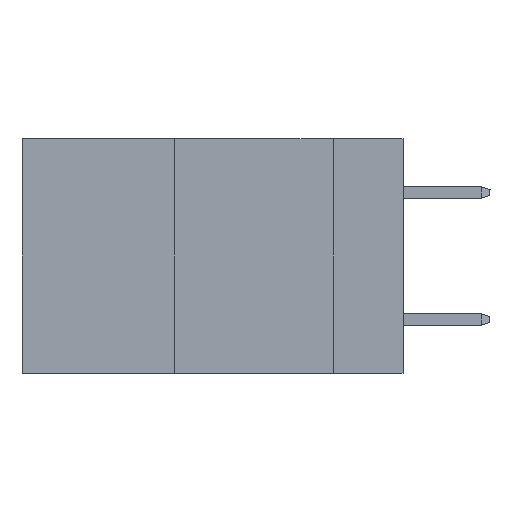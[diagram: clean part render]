
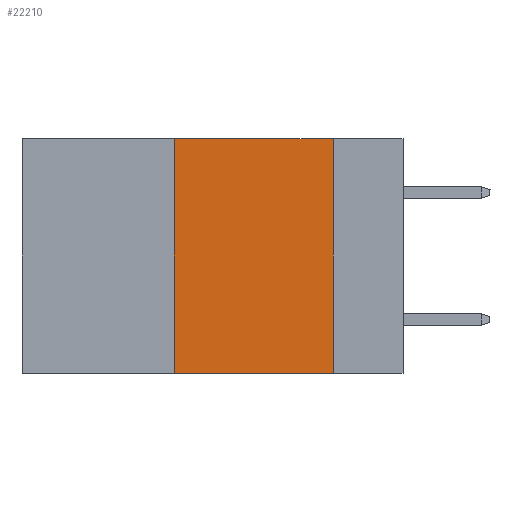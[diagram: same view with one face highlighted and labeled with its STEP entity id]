
A CAD part, left-side view. The second image highlights one B-rep face of the part: STEP entity #22210.
In plain terms, the highlighted planar face has unit normal (-1, 0, 0).
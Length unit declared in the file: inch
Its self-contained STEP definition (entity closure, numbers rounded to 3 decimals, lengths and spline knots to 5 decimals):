
#9 = CARTESIAN_POINT ( 'NONE',  ( 0., 0.11, 0. ) ) ;
#233 = EDGE_CURVE ( 'NONE', #37022, #9267, #14682, .T. ) ;
#369 = CARTESIAN_POINT ( 'NONE',  ( 0., 0.36, -0.37 ) ) ;
#1321 = ORIENTED_EDGE ( 'NONE', *, *, #233, .F. ) ;
#2073 = LINE ( 'NONE', #17226, #29607 ) ;
#2598 = EDGE_CURVE ( 'NONE', #9267, #5911, #8697, .T. ) ;
#5911 = VERTEX_POINT ( 'NONE', #25735 ) ;
#6318 = DIRECTION ( 'NONE',  ( 0., 0., -1. ) ) ;
#6569 = DIRECTION ( 'NONE',  ( 0., -1., 0. ) ) ;
#7656 = EDGE_CURVE ( 'NONE', #36403, #37022, #2073, .T. ) ;
#8594 = VECTOR ( 'NONE', #23567, 39.37008 ) ;
#8697 = LINE ( 'NONE', #9, #31624 ) ;
#9267 = VERTEX_POINT ( 'NONE', #36889 ) ;
#14262 = EDGE_CURVE ( 'NONE', #36403, #5911, #27625, .T. ) ;
#14682 = LINE ( 'NONE', #29279, #8594 ) ;
#15802 = CARTESIAN_POINT ( 'NONE',  ( 0., 0.6, -0.37 ) ) ;
#17226 = CARTESIAN_POINT ( 'NONE',  ( 0., 0.36, 0. ) ) ;
#18154 = DIRECTION ( 'NONE',  ( 1., 0., 0. ) ) ;
#19775 = VECTOR ( 'NONE', #6569, 39.37008 ) ;
#19960 = ORIENTED_EDGE ( 'NONE', *, *, #14262, .T. ) ;
#21121 = DIRECTION ( 'NONE',  ( 0., 0., -1. ) ) ;
#22210 = ADVANCED_FACE ( 'NONE', ( #32955 ), #35915, .F. ) ;
#23567 = DIRECTION ( 'NONE',  ( 0., -1., 0. ) ) ;
#23874 = CARTESIAN_POINT ( 'NONE',  ( 0., 0.6, 0. ) ) ;
#25735 = CARTESIAN_POINT ( 'NONE',  ( 0., 0.11, -0.37 ) ) ;
#26541 = EDGE_LOOP ( 'NONE', ( #36272, #1321, #32516, #19960 ) ) ;
#27625 = LINE ( 'NONE', #15802, #19775 ) ;
#29257 = DIRECTION ( 'NONE',  ( 0., 0., 1. ) ) ;
#29279 = CARTESIAN_POINT ( 'NONE',  ( 0., 0.6, 0. ) ) ;
#29607 = VECTOR ( 'NONE', #29257, 39.37008 ) ;
#31624 = VECTOR ( 'NONE', #6318, 39.37008 ) ;
#32516 = ORIENTED_EDGE ( 'NONE', *, *, #7656, .F. ) ;
#32955 = FACE_OUTER_BOUND ( 'NONE', #26541, .T. ) ;
#35370 = AXIS2_PLACEMENT_3D ( 'NONE', #23874, #18154, #21121 ) ;
#35915 = PLANE ( 'NONE',  #35370 ) ;
#36272 = ORIENTED_EDGE ( 'NONE', *, *, #2598, .F. ) ;
#36403 = VERTEX_POINT ( 'NONE', #369 ) ;
#36889 = CARTESIAN_POINT ( 'NONE',  ( 0., 0.11, 0. ) ) ;
#37022 = VERTEX_POINT ( 'NONE', #38101 ) ;
#38101 = CARTESIAN_POINT ( 'NONE',  ( 0., 0.36, 0. ) ) ;
